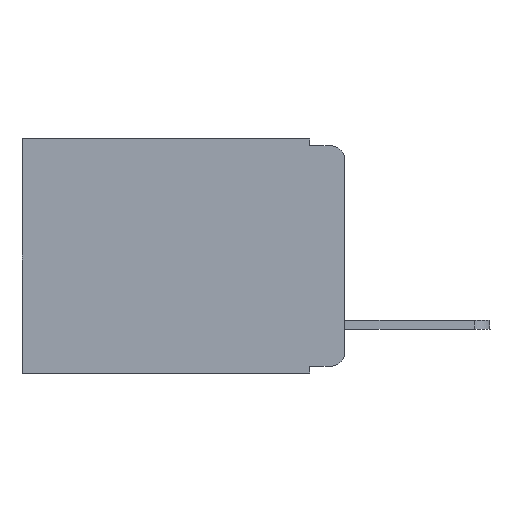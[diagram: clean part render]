
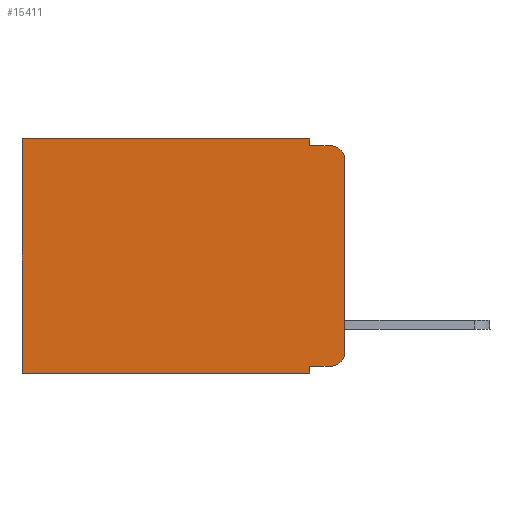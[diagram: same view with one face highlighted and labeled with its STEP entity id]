
A CAD part, left-side view. The second image highlights one B-rep face of the part: STEP entity #15411.
In plain terms, the highlighted planar face has unit normal (-1, 0, 0).
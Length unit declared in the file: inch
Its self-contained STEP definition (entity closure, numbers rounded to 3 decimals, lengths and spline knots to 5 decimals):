
#503 = EDGE_CURVE ( 'NONE', #11584, #6098, #20396, .T. ) ;
#579 = AXIS2_PLACEMENT_3D ( 'NONE', #17329, #13207, #20704 ) ;
#1081 = DIRECTION ( 'NONE',  ( 0., 0., -1. ) ) ;
#1792 = AXIS2_PLACEMENT_3D ( 'NONE', #11090, #20574, #1081 ) ;
#1870 = CARTESIAN_POINT ( 'NONE',  ( 0.298, 0.051, -0.01 ) ) ;
#1908 = VECTOR ( 'NONE', #24562, 39.37008 ) ;
#1969 = CARTESIAN_POINT ( 'NONE',  ( 0.298, 0.051, -0.333 ) ) ;
#2240 = DIRECTION ( 'NONE',  ( 0., 0., -1. ) ) ;
#2582 = EDGE_CURVE ( 'NONE', #17684, #14625, #9334, .T. ) ;
#3171 = CIRCLE ( 'NONE', #15155, 0.02 ) ;
#3222 = ORIENTED_EDGE ( 'NONE', *, *, #22207, .F. ) ;
#3326 = VECTOR ( 'NONE', #11348, 39.37008 ) ;
#3635 = ORIENTED_EDGE ( 'NONE', *, *, #13578, .F. ) ;
#3708 = CARTESIAN_POINT ( 'NONE',  ( 0.298, 0., -0.343 ) ) ;
#4684 = LINE ( 'NONE', #8688, #23478 ) ;
#5153 = ORIENTED_EDGE ( 'NONE', *, *, #9384, .T. ) ;
#5342 = EDGE_CURVE ( 'NONE', #22424, #17775, #15336, .T. ) ;
#5583 = LINE ( 'NONE', #3708, #3326 ) ;
#5997 = CARTESIAN_POINT ( 'NONE',  ( 0.298, 0.051, 0. ) ) ;
#6098 = VERTEX_POINT ( 'NONE', #20395 ) ;
#7003 = CARTESIAN_POINT ( 'NONE',  ( 0.298, 0., -0.313 ) ) ;
#7490 = ORIENTED_EDGE ( 'NONE', *, *, #2582, .F. ) ;
#7495 = CARTESIAN_POINT ( 'NONE',  ( 0.298, 0.02, -0.333 ) ) ;
#7501 = CARTESIAN_POINT ( 'NONE',  ( 0.298, 0.02, -0.313 ) ) ;
#7681 = VECTOR ( 'NONE', #12365, 39.37008 ) ;
#7862 = LINE ( 'NONE', #13878, #18748 ) ;
#8005 = CARTESIAN_POINT ( 'NONE',  ( 0.298, 0.473, -0.343 ) ) ;
#8115 = CARTESIAN_POINT ( 'NONE',  ( 0.298, 0., 0. ) ) ;
#8688 = CARTESIAN_POINT ( 'NONE',  ( 0.298, 0.051, 0. ) ) ;
#9035 = VERTEX_POINT ( 'NONE', #8005 ) ;
#9205 = FACE_OUTER_BOUND ( 'NONE', #18731, .T. ) ;
#9334 = LINE ( 'NONE', #24450, #12618 ) ;
#9384 = EDGE_CURVE ( 'NONE', #23789, #14625, #10171, .T. ) ;
#9503 = DIRECTION ( 'NONE',  ( 0., 0., -1. ) ) ;
#9951 = CARTESIAN_POINT ( 'NONE',  ( 0.298, 0.051, -0.333 ) ) ;
#10171 = CIRCLE ( 'NONE', #579, 0.02 ) ;
#11090 = CARTESIAN_POINT ( 'NONE',  ( 0.298, 0., 0. ) ) ;
#11237 = VECTOR ( 'NONE', #17340, 39.37008 ) ;
#11348 = DIRECTION ( 'NONE',  ( 0., 1., 0. ) ) ;
#11584 = VERTEX_POINT ( 'NONE', #5997 ) ;
#11913 = CARTESIAN_POINT ( 'NONE',  ( 0.298, 0.051, -0.343 ) ) ;
#12365 = DIRECTION ( 'NONE',  ( 0., 0., -1. ) ) ;
#12618 = VECTOR ( 'NONE', #13209, 39.37008 ) ;
#13207 = DIRECTION ( 'NONE',  ( -1., 0., 0. ) ) ;
#13209 = DIRECTION ( 'NONE',  ( 0., -1., 0. ) ) ;
#13578 = EDGE_CURVE ( 'NONE', #23789, #23081, #16111, .T. ) ;
#13878 = CARTESIAN_POINT ( 'NONE',  ( 0.298, 0.051, 0. ) ) ;
#14560 = ORIENTED_EDGE ( 'NONE', *, *, #22525, .F. ) ;
#14625 = VERTEX_POINT ( 'NONE', #22376 ) ;
#14924 = CARTESIAN_POINT ( 'NONE',  ( 0.298, 0., 0. ) ) ;
#15155 = AXIS2_PLACEMENT_3D ( 'NONE', #7501, #16881, #9503 ) ;
#15336 = LINE ( 'NONE', #9951, #11237 ) ;
#15411 = ADVANCED_FACE ( 'NONE', ( #9205 ), #22059, .F. ) ;
#16111 = LINE ( 'NONE', #8115, #7681 ) ;
#16117 = VERTEX_POINT ( 'NONE', #11913 ) ;
#16881 = DIRECTION ( 'NONE',  ( -1., 0., 0. ) ) ;
#17329 = CARTESIAN_POINT ( 'NONE',  ( 0.298, 0.02, -0.03 ) ) ;
#17340 = DIRECTION ( 'NONE',  ( 0., -1., 0. ) ) ;
#17684 = VERTEX_POINT ( 'NONE', #1870 ) ;
#17711 = VECTOR ( 'NONE', #22646, 39.37008 ) ;
#17775 = VERTEX_POINT ( 'NONE', #7495 ) ;
#18330 = ORIENTED_EDGE ( 'NONE', *, *, #19923, .T. ) ;
#18731 = EDGE_LOOP ( 'NONE', ( #3635, #5153, #7490, #19984, #21869, #18330, #14560, #3222, #21025, #20443 ) ) ;
#18748 = VECTOR ( 'NONE', #2240, 39.37008 ) ;
#19923 = EDGE_CURVE ( 'NONE', #6098, #9035, #22920, .T. ) ;
#19984 = ORIENTED_EDGE ( 'NONE', *, *, #20833, .F. ) ;
#20395 = CARTESIAN_POINT ( 'NONE',  ( 0.298, 0.473, 0. ) ) ;
#20396 = LINE ( 'NONE', #14924, #17711 ) ;
#20443 = ORIENTED_EDGE ( 'NONE', *, *, #21990, .T. ) ;
#20574 = DIRECTION ( 'NONE',  ( 1., 0., 0. ) ) ;
#20704 = DIRECTION ( 'NONE',  ( 0., 0., -1. ) ) ;
#20833 = EDGE_CURVE ( 'NONE', #11584, #17684, #4684, .T. ) ;
#21025 = ORIENTED_EDGE ( 'NONE', *, *, #5342, .T. ) ;
#21869 = ORIENTED_EDGE ( 'NONE', *, *, #503, .T. ) ;
#21990 = EDGE_CURVE ( 'NONE', #17775, #23081, #3171, .T. ) ;
#22059 = PLANE ( 'NONE',  #1792 ) ;
#22207 = EDGE_CURVE ( 'NONE', #22424, #16117, #7862, .T. ) ;
#22376 = CARTESIAN_POINT ( 'NONE',  ( 0.298, 0.02, -0.01 ) ) ;
#22424 = VERTEX_POINT ( 'NONE', #1969 ) ;
#22525 = EDGE_CURVE ( 'NONE', #16117, #9035, #5583, .T. ) ;
#22646 = DIRECTION ( 'NONE',  ( 0., 1., 0. ) ) ;
#22828 = CARTESIAN_POINT ( 'NONE',  ( 0.298, 0., -0.03 ) ) ;
#22920 = LINE ( 'NONE', #23046, #1908 ) ;
#23046 = CARTESIAN_POINT ( 'NONE',  ( 0.298, 0.473, 0. ) ) ;
#23081 = VERTEX_POINT ( 'NONE', #7003 ) ;
#23440 = DIRECTION ( 'NONE',  ( 0., 0., -1. ) ) ;
#23478 = VECTOR ( 'NONE', #23440, 39.37008 ) ;
#23789 = VERTEX_POINT ( 'NONE', #22828 ) ;
#24450 = CARTESIAN_POINT ( 'NONE',  ( 0.298, 0.051, -0.01 ) ) ;
#24562 = DIRECTION ( 'NONE',  ( 0., 0., -1. ) ) ;
